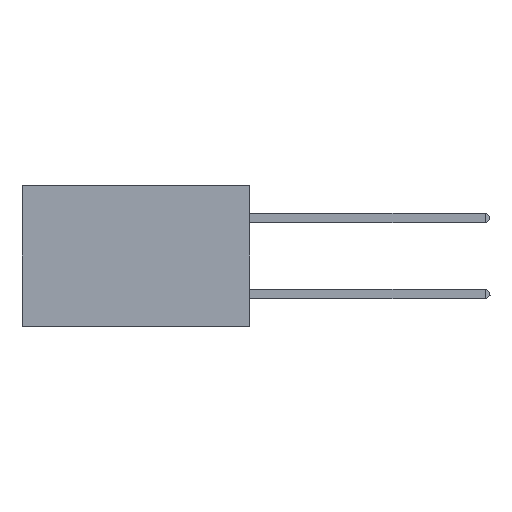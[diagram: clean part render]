
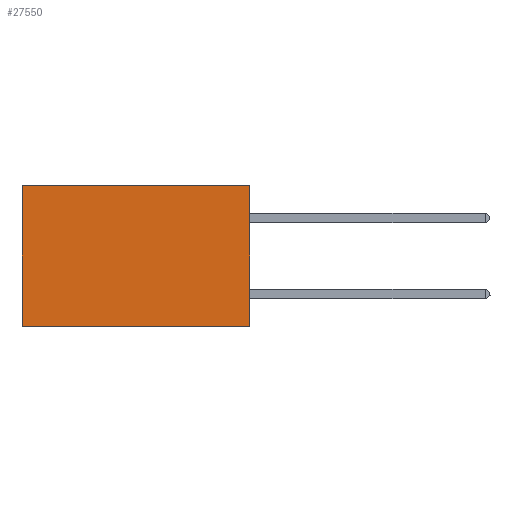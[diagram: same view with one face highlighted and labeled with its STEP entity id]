
A CAD part, left-side view. The second image highlights one B-rep face of the part: STEP entity #27550.
In plain terms, the highlighted planar face has unit normal (-1, 0, 0).
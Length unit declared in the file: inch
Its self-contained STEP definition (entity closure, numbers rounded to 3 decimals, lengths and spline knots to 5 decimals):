
#236 = DIRECTION ( 'NONE',  ( 0., 1., 0. ) ) ;
#393 = ORIENTED_EDGE ( 'NONE', *, *, #8995, .T. ) ;
#1292 = CARTESIAN_POINT ( 'NONE',  ( 0.2875, 0.6, -0.37 ) ) ;
#1474 = CARTESIAN_POINT ( 'NONE',  ( 0.2875, 0., -0.37 ) ) ;
#2772 = EDGE_LOOP ( 'NONE', ( #393, #10797, #6510, #7607 ) ) ;
#3397 = CARTESIAN_POINT ( 'NONE',  ( 0.2875, 0., -0.37 ) ) ;
#4616 = PLANE ( 'NONE',  #29276 ) ;
#4944 = VERTEX_POINT ( 'NONE', #1474 ) ;
#5718 = DIRECTION ( 'NONE',  ( 0., 1., 0. ) ) ;
#6510 = ORIENTED_EDGE ( 'NONE', *, *, #13622, .F. ) ;
#7607 = ORIENTED_EDGE ( 'NONE', *, *, #11758, .T. ) ;
#8995 = EDGE_CURVE ( 'NONE', #28427, #16862, #25680, .T. ) ;
#9683 = CARTESIAN_POINT ( 'NONE',  ( 0.2875, 0., 0. ) ) ;
#10237 = CARTESIAN_POINT ( 'NONE',  ( 0.2875, 0., 0. ) ) ;
#10797 = ORIENTED_EDGE ( 'NONE', *, *, #26587, .F. ) ;
#11758 = EDGE_CURVE ( 'NONE', #28238, #28427, #29439, .T. ) ;
#13622 = EDGE_CURVE ( 'NONE', #28238, #4944, #14788, .T. ) ;
#13955 = CARTESIAN_POINT ( 'NONE',  ( 0.2875, 0.6, 0. ) ) ;
#14055 = DIRECTION ( 'NONE',  ( 0., 0., -1. ) ) ;
#14738 = CARTESIAN_POINT ( 'NONE',  ( 0.2875, 0., 0. ) ) ;
#14788 = LINE ( 'NONE', #9683, #19099 ) ;
#16862 = VERTEX_POINT ( 'NONE', #1292 ) ;
#18958 = VECTOR ( 'NONE', #14055, 39.37008 ) ;
#19099 = VECTOR ( 'NONE', #29662, 39.37008 ) ;
#20327 = VECTOR ( 'NONE', #236, 39.37008 ) ;
#20635 = CARTESIAN_POINT ( 'NONE',  ( 0.2875, 0., 0. ) ) ;
#20885 = CARTESIAN_POINT ( 'NONE',  ( 0.2875, 0.6, 0. ) ) ;
#21007 = FACE_OUTER_BOUND ( 'NONE', #2772, .T. ) ;
#21888 = VECTOR ( 'NONE', #5718, 39.37008 ) ;
#22715 = DIRECTION ( 'NONE',  ( 0., 0., -1. ) ) ;
#25680 = LINE ( 'NONE', #13955, #18958 ) ;
#26587 = EDGE_CURVE ( 'NONE', #4944, #16862, #29022, .T. ) ;
#27550 = ADVANCED_FACE ( 'NONE', ( #21007 ), #4616, .F. ) ;
#28238 = VERTEX_POINT ( 'NONE', #14738 ) ;
#28427 = VERTEX_POINT ( 'NONE', #20885 ) ;
#29022 = LINE ( 'NONE', #3397, #21888 ) ;
#29276 = AXIS2_PLACEMENT_3D ( 'NONE', #20635, #32525, #22715 ) ;
#29439 = LINE ( 'NONE', #10237, #20327 ) ;
#29662 = DIRECTION ( 'NONE',  ( 0., 0., -1. ) ) ;
#32525 = DIRECTION ( 'NONE',  ( 1., 0., 0. ) ) ;
